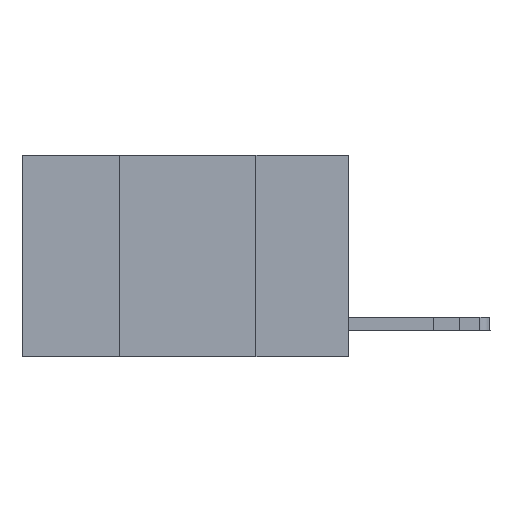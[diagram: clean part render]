
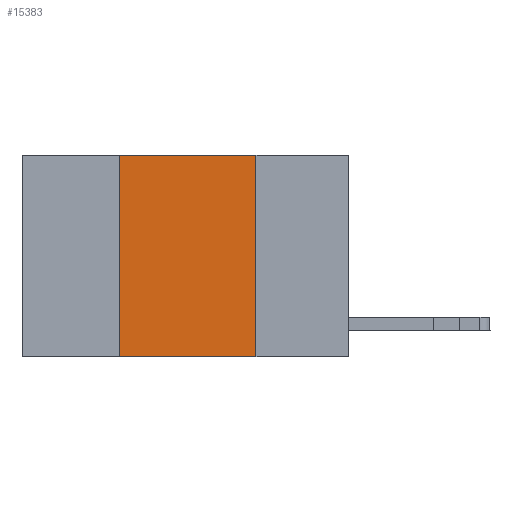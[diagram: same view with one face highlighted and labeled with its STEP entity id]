
A CAD part, left-side view. The second image highlights one B-rep face of the part: STEP entity #15383.
In plain terms, the highlighted planar face has unit normal (-1, 0, 0).
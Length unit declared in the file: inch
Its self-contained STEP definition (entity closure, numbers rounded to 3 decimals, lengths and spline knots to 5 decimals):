
#919 = VERTEX_POINT ( 'NONE', #8305 ) ;
#1268 = EDGE_CURVE ( 'NONE', #4074, #3347, #14266, .T. ) ;
#1544 = ORIENTED_EDGE ( 'NONE', *, *, #3804, .F. ) ;
#1968 = EDGE_CURVE ( 'NONE', #4074, #919, #5374, .T. ) ;
#2026 = VECTOR ( 'NONE', #8981, 39.37008 ) ;
#2177 = ORIENTED_EDGE ( 'NONE', *, *, #2878, .F. ) ;
#2867 = CARTESIAN_POINT ( 'NONE',  ( 0., 0.6, -0.37 ) ) ;
#2878 = EDGE_CURVE ( 'NONE', #919, #5999, #3211, .T. ) ;
#3211 = LINE ( 'NONE', #5663, #8865 ) ;
#3347 = VERTEX_POINT ( 'NONE', #14715 ) ;
#3793 = DIRECTION ( 'NONE',  ( 1., 0., 0. ) ) ;
#3804 = EDGE_CURVE ( 'NONE', #5999, #3347, #8465, .T. ) ;
#4074 = VERTEX_POINT ( 'NONE', #8984 ) ;
#4784 = CARTESIAN_POINT ( 'NONE',  ( 0., 0.17, 0. ) ) ;
#4962 = CARTESIAN_POINT ( 'NONE',  ( 0., 0.17, 0. ) ) ;
#5335 = DIRECTION ( 'NONE',  ( 0., -1., 0. ) ) ;
#5374 = LINE ( 'NONE', #12513, #2026 ) ;
#5663 = CARTESIAN_POINT ( 'NONE',  ( 0., 0.6, 0. ) ) ;
#5999 = VERTEX_POINT ( 'NONE', #4784 ) ;
#6199 = ORIENTED_EDGE ( 'NONE', *, *, #1968, .F. ) ;
#8000 = VECTOR ( 'NONE', #5335, 39.37008 ) ;
#8305 = CARTESIAN_POINT ( 'NONE',  ( 0., 0.42, 0. ) ) ;
#8435 = EDGE_LOOP ( 'NONE', ( #1544, #2177, #6199, #12318 ) ) ;
#8465 = LINE ( 'NONE', #4962, #14015 ) ;
#8578 = PLANE ( 'NONE',  #9857 ) ;
#8865 = VECTOR ( 'NONE', #13933, 39.37008 ) ;
#8981 = DIRECTION ( 'NONE',  ( 0., 0., 1. ) ) ;
#8984 = CARTESIAN_POINT ( 'NONE',  ( 0., 0.42, -0.37 ) ) ;
#9749 = CARTESIAN_POINT ( 'NONE',  ( 0., 0.6, 0. ) ) ;
#9857 = AXIS2_PLACEMENT_3D ( 'NONE', #9749, #3793, #12143 ) ;
#12052 = DIRECTION ( 'NONE',  ( 0., 0., -1. ) ) ;
#12143 = DIRECTION ( 'NONE',  ( 0., 0., -1. ) ) ;
#12318 = ORIENTED_EDGE ( 'NONE', *, *, #1268, .T. ) ;
#12513 = CARTESIAN_POINT ( 'NONE',  ( 0., 0.42, 0. ) ) ;
#13100 = FACE_OUTER_BOUND ( 'NONE', #8435, .T. ) ;
#13933 = DIRECTION ( 'NONE',  ( 0., -1., 0. ) ) ;
#14015 = VECTOR ( 'NONE', #12052, 39.37008 ) ;
#14266 = LINE ( 'NONE', #2867, #8000 ) ;
#14715 = CARTESIAN_POINT ( 'NONE',  ( 0., 0.17, -0.37 ) ) ;
#15383 = ADVANCED_FACE ( 'NONE', ( #13100 ), #8578, .F. ) ;
